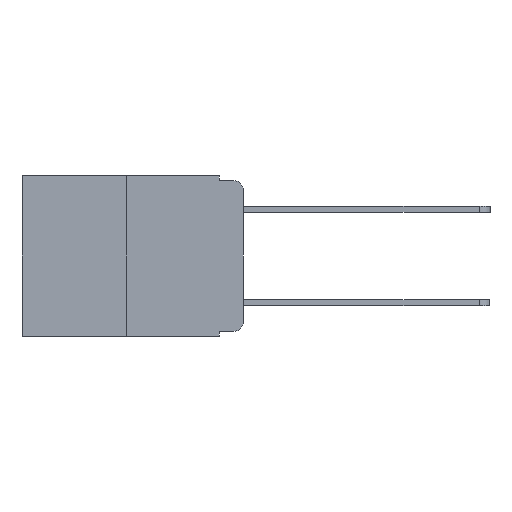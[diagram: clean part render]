
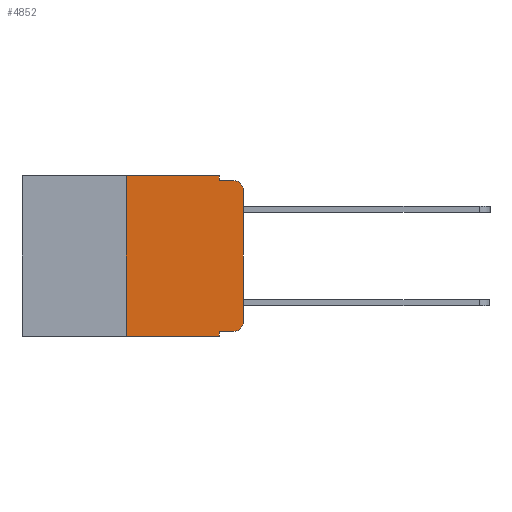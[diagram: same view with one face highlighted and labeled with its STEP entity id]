
A CAD part, left-side view. The second image highlights one B-rep face of the part: STEP entity #4852.
In plain terms, the highlighted planar face has unit normal (-1, 0, 0).
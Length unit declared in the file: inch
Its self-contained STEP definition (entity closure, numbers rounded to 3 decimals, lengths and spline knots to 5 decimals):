
#102 = DIRECTION ( 'NONE',  ( 1., 0., 0. ) ) ;
#200 = CARTESIAN_POINT ( 'NONE',  ( 0., 0.051, -0.333 ) ) ;
#258 = CARTESIAN_POINT ( 'NONE',  ( 0., 0.25, 0. ) ) ;
#521 = VECTOR ( 'NONE', #780, 39.37008 ) ;
#780 = DIRECTION ( 'NONE',  ( 0., -1., 0. ) ) ;
#789 = VECTOR ( 'NONE', #1365, 39.37008 ) ;
#1021 = ORIENTED_EDGE ( 'NONE', *, *, #3756, .F. ) ;
#1045 = LINE ( 'NONE', #1391, #8519 ) ;
#1170 = VERTEX_POINT ( 'NONE', #1877 ) ;
#1308 = DIRECTION ( 'NONE',  ( -1., 0., 0. ) ) ;
#1363 = CARTESIAN_POINT ( 'NONE',  ( 0., 0.02, -0.03 ) ) ;
#1365 = DIRECTION ( 'NONE',  ( 0., -1., 0. ) ) ;
#1391 = CARTESIAN_POINT ( 'NONE',  ( 0., 0.051, 0. ) ) ;
#1420 = CARTESIAN_POINT ( 'NONE',  ( 0., 0.25, 0. ) ) ;
#1663 = ORIENTED_EDGE ( 'NONE', *, *, #5163, .F. ) ;
#1877 = CARTESIAN_POINT ( 'NONE',  ( 0., 0., -0.313 ) ) ;
#1906 = VECTOR ( 'NONE', #10948, 39.37008 ) ;
#1934 = CARTESIAN_POINT ( 'NONE',  ( 0., 0.051, -0.01 ) ) ;
#2149 = VERTEX_POINT ( 'NONE', #10179 ) ;
#2348 = CARTESIAN_POINT ( 'NONE',  ( 0., 0., 0. ) ) ;
#2441 = ORIENTED_EDGE ( 'NONE', *, *, #4826, .T. ) ;
#2514 = ORIENTED_EDGE ( 'NONE', *, *, #5236, .T. ) ;
#2675 = ORIENTED_EDGE ( 'NONE', *, *, #4942, .F. ) ;
#2686 = DIRECTION ( 'NONE',  ( 0., 0., -1. ) ) ;
#3208 = CARTESIAN_POINT ( 'NONE',  ( 0., 0.473, 0. ) ) ;
#3280 = AXIS2_PLACEMENT_3D ( 'NONE', #1363, #1308, #8694 ) ;
#3326 = ORIENTED_EDGE ( 'NONE', *, *, #5500, .T. ) ;
#3367 = DIRECTION ( 'NONE',  ( 0., -1., 0. ) ) ;
#3377 = VERTEX_POINT ( 'NONE', #258 ) ;
#3540 = LINE ( 'NONE', #9314, #521 ) ;
#3646 = VERTEX_POINT ( 'NONE', #5221 ) ;
#3687 = ORIENTED_EDGE ( 'NONE', *, *, #5548, .F. ) ;
#3756 = EDGE_CURVE ( 'NONE', #3377, #8920, #6790, .T. ) ;
#4040 = CARTESIAN_POINT ( 'NONE',  ( 0., 0.051, -0.333 ) ) ;
#4826 = EDGE_CURVE ( 'NONE', #3646, #2149, #3540, .T. ) ;
#4852 = ADVANCED_FACE ( 'NONE', ( #12262 ), #5335, .F. ) ;
#4942 = EDGE_CURVE ( 'NONE', #8174, #2149, #1045, .T. ) ;
#5095 = DIRECTION ( 'NONE',  ( 0., 0., -1. ) ) ;
#5163 = EDGE_CURVE ( 'NONE', #3646, #3377, #9803, .T. ) ;
#5202 = LINE ( 'NONE', #8878, #1906 ) ;
#5221 = CARTESIAN_POINT ( 'NONE',  ( 0., 0.25, -0.343 ) ) ;
#5223 = ORIENTED_EDGE ( 'NONE', *, *, #5507, .T. ) ;
#5236 = EDGE_CURVE ( 'NONE', #8174, #10497, #10185, .T. ) ;
#5335 = PLANE ( 'NONE',  #6145 ) ;
#5500 = EDGE_CURVE ( 'NONE', #1170, #10222, #5845, .T. ) ;
#5507 = EDGE_CURVE ( 'NONE', #10222, #11910, #7942, .T. ) ;
#5529 = EDGE_CURVE ( 'NONE', #8284, #11910, #9923, .T. ) ;
#5548 = EDGE_CURVE ( 'NONE', #8920, #8284, #5202, .T. ) ;
#5813 = AXIS2_PLACEMENT_3D ( 'NONE', #6584, #10404, #5095 ) ;
#5845 = LINE ( 'NONE', #2348, #10181 ) ;
#6145 = AXIS2_PLACEMENT_3D ( 'NONE', #3208, #102, #12010 ) ;
#6584 = CARTESIAN_POINT ( 'NONE',  ( 0., 0.02, -0.313 ) ) ;
#6650 = CARTESIAN_POINT ( 'NONE',  ( 0., 0.473, 0. ) ) ;
#6790 = LINE ( 'NONE', #6650, #789 ) ;
#6813 = CARTESIAN_POINT ( 'NONE',  ( 0., 0.02, -0.01 ) ) ;
#7234 = EDGE_CURVE ( 'NONE', #10497, #1170, #9637, .T. ) ;
#7247 = CARTESIAN_POINT ( 'NONE',  ( 0., 0.02, -0.333 ) ) ;
#7394 = VECTOR ( 'NONE', #9636, 39.37008 ) ;
#7942 = CIRCLE ( 'NONE', #3280, 0.02 ) ;
#7947 = VECTOR ( 'NONE', #3367, 39.37008 ) ;
#8174 = VERTEX_POINT ( 'NONE', #4040 ) ;
#8284 = VERTEX_POINT ( 'NONE', #9414 ) ;
#8519 = VECTOR ( 'NONE', #2686, 39.37008 ) ;
#8694 = DIRECTION ( 'NONE',  ( 0., 0., -1. ) ) ;
#8878 = CARTESIAN_POINT ( 'NONE',  ( 0., 0.051, 0. ) ) ;
#8920 = VERTEX_POINT ( 'NONE', #9019 ) ;
#9019 = CARTESIAN_POINT ( 'NONE',  ( 0., 0.051, 0. ) ) ;
#9083 = ORIENTED_EDGE ( 'NONE', *, *, #5529, .F. ) ;
#9314 = CARTESIAN_POINT ( 'NONE',  ( 0., 0.473, -0.343 ) ) ;
#9414 = CARTESIAN_POINT ( 'NONE',  ( 0., 0.051, -0.01 ) ) ;
#9456 = ORIENTED_EDGE ( 'NONE', *, *, #7234, .T. ) ;
#9636 = DIRECTION ( 'NONE',  ( 0., -1., 0. ) ) ;
#9637 = CIRCLE ( 'NONE', #5813, 0.02 ) ;
#9803 = LINE ( 'NONE', #1420, #11473 ) ;
#9923 = LINE ( 'NONE', #1934, #7394 ) ;
#10179 = CARTESIAN_POINT ( 'NONE',  ( 0., 0.051, -0.343 ) ) ;
#10181 = VECTOR ( 'NONE', #11070, 39.37008 ) ;
#10185 = LINE ( 'NONE', #200, #7947 ) ;
#10222 = VERTEX_POINT ( 'NONE', #11016 ) ;
#10404 = DIRECTION ( 'NONE',  ( -1., 0., 0. ) ) ;
#10497 = VERTEX_POINT ( 'NONE', #7247 ) ;
#10948 = DIRECTION ( 'NONE',  ( 0., 0., -1. ) ) ;
#11016 = CARTESIAN_POINT ( 'NONE',  ( 0., 0., -0.03 ) ) ;
#11070 = DIRECTION ( 'NONE',  ( 0., 0., 1. ) ) ;
#11100 = EDGE_LOOP ( 'NONE', ( #3326, #5223, #9083, #3687, #1021, #1663, #2441, #2675, #2514, #9456 ) ) ;
#11312 = DIRECTION ( 'NONE',  ( 0., 0., 1. ) ) ;
#11473 = VECTOR ( 'NONE', #11312, 39.37008 ) ;
#11910 = VERTEX_POINT ( 'NONE', #6813 ) ;
#12010 = DIRECTION ( 'NONE',  ( 0., 0., -1. ) ) ;
#12262 = FACE_OUTER_BOUND ( 'NONE', #11100, .T. ) ;
